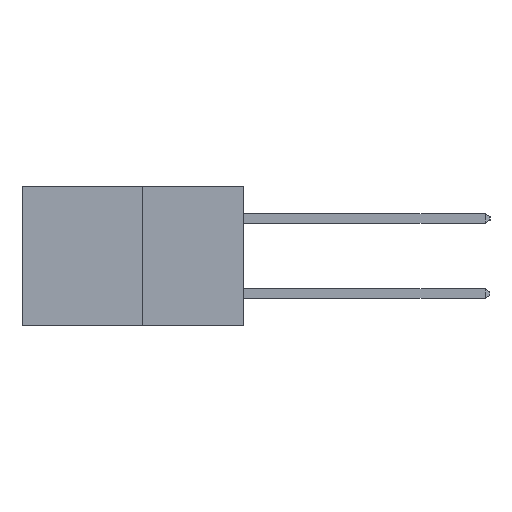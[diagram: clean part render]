
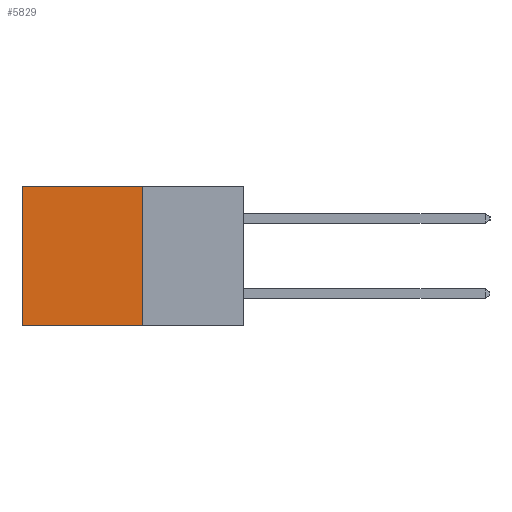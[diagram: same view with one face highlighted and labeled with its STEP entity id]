
A CAD part, left-side view. The second image highlights one B-rep face of the part: STEP entity #5829.
In plain terms, the highlighted planar face has unit normal (-1, 0, 0).
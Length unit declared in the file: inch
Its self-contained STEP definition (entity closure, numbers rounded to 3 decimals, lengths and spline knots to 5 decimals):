
#6 = VERTEX_POINT ( 'NONE', #3289 ) ;
#1324 = VECTOR ( 'NONE', #15546, 39.37008 ) ;
#1588 = VECTOR ( 'NONE', #4727, 39.37008 ) ;
#1978 = AXIS2_PLACEMENT_3D ( 'NONE', #6221, #9696, #21326 ) ;
#2536 = LINE ( 'NONE', #3213, #20056 ) ;
#3213 = CARTESIAN_POINT ( 'NONE',  ( 0.277, 0.59, -0.37 ) ) ;
#3289 = CARTESIAN_POINT ( 'NONE',  ( 0.277, 0.27, 0. ) ) ;
#3717 = VERTEX_POINT ( 'NONE', #5171 ) ;
#4727 = DIRECTION ( 'NONE',  ( 0., 0., -1. ) ) ;
#5171 = CARTESIAN_POINT ( 'NONE',  ( 0.277, 0.59, -0.37 ) ) ;
#5203 = EDGE_CURVE ( 'NONE', #6, #9948, #6806, .T. ) ;
#5420 = ORIENTED_EDGE ( 'NONE', *, *, #16121, .T. ) ;
#5829 = ADVANCED_FACE ( 'NONE', ( #11605 ), #14736, .F. ) ;
#5992 = ORIENTED_EDGE ( 'NONE', *, *, #5203, .F. ) ;
#6221 = CARTESIAN_POINT ( 'NONE',  ( 0.277, 0.27, -0.37 ) ) ;
#6806 = LINE ( 'NONE', #11590, #1588 ) ;
#8497 = CARTESIAN_POINT ( 'NONE',  ( 0.277, 0.27, -0.37 ) ) ;
#8681 = EDGE_LOOP ( 'NONE', ( #18330, #20332, #5992, #5420 ) ) ;
#9696 = DIRECTION ( 'NONE',  ( 1., 0., 0. ) ) ;
#9754 = DIRECTION ( 'NONE',  ( 0., 0., -1. ) ) ;
#9948 = VERTEX_POINT ( 'NONE', #8497 ) ;
#11590 = CARTESIAN_POINT ( 'NONE',  ( 0.277, 0.27, -0.37 ) ) ;
#11605 = FACE_OUTER_BOUND ( 'NONE', #8681, .T. ) ;
#12117 = VERTEX_POINT ( 'NONE', #13085 ) ;
#12204 = CARTESIAN_POINT ( 'NONE',  ( 0.277, 0.27, -0.37 ) ) ;
#13085 = CARTESIAN_POINT ( 'NONE',  ( 0.277, 0.59, 0. ) ) ;
#13385 = LINE ( 'NONE', #12204, #17242 ) ;
#13753 = EDGE_CURVE ( 'NONE', #12117, #3717, #2536, .T. ) ;
#13890 = DIRECTION ( 'NONE',  ( 0., 1., 0. ) ) ;
#14736 = PLANE ( 'NONE',  #1978 ) ;
#15051 = LINE ( 'NONE', #18808, #1324 ) ;
#15546 = DIRECTION ( 'NONE',  ( 0., 1., 0. ) ) ;
#16121 = EDGE_CURVE ( 'NONE', #6, #12117, #15051, .T. ) ;
#17242 = VECTOR ( 'NONE', #13890, 39.37008 ) ;
#18330 = ORIENTED_EDGE ( 'NONE', *, *, #13753, .T. ) ;
#18808 = CARTESIAN_POINT ( 'NONE',  ( 0.277, 0.27, 0. ) ) ;
#20056 = VECTOR ( 'NONE', #9754, 39.37008 ) ;
#20332 = ORIENTED_EDGE ( 'NONE', *, *, #21425, .F. ) ;
#21326 = DIRECTION ( 'NONE',  ( 0., 0., -1. ) ) ;
#21425 = EDGE_CURVE ( 'NONE', #9948, #3717, #13385, .T. ) ;
